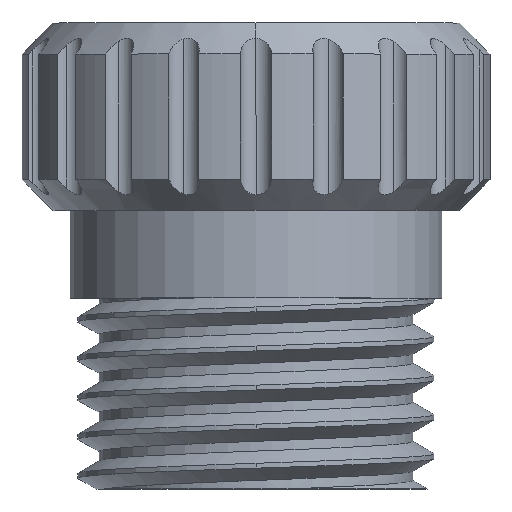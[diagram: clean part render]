
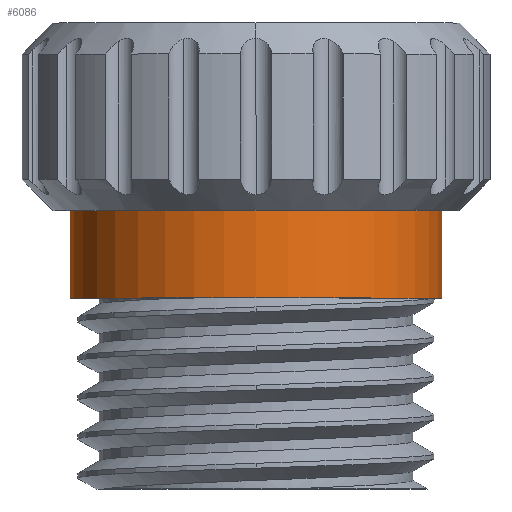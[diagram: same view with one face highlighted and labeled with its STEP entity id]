
A CAD part, top view. The second image highlights one B-rep face of the part: STEP entity #6086.
In plain terms, the highlighted cylindrical face has radius 7.556 mm (diameter 15.113 mm), a partial arc.
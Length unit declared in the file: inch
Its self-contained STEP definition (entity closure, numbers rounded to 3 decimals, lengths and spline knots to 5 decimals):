
#25 = DIRECTION ( 'NONE',  ( 0., -1., 0. ) ) ;
#44 = EDGE_CURVE ( 'NONE', #6907, #3247, #344, .T. ) ;
#344 = CIRCLE ( 'NONE', #1321, 0.2975 ) ;
#438 = CARTESIAN_POINT ( 'NONE',  ( 0., 0.305, -0.09256 ) ) ;
#463 = CARTESIAN_POINT ( 'NONE',  ( 0.16126, 0.305, -0.34256 ) ) ;
#691 = VECTOR ( 'NONE', #1452, 39.37008 ) ;
#1013 = ORIENTED_EDGE ( 'NONE', *, *, #2857, .T. ) ;
#1178 = DIRECTION ( 'NONE',  ( 0., 0., 1. ) ) ;
#1321 = AXIS2_PLACEMENT_3D ( 'NONE', #5092, #25, #1178 ) ;
#1392 = CARTESIAN_POINT ( 'NONE',  ( -0.16126, 0.305, -0.34256 ) ) ;
#1452 = DIRECTION ( 'NONE',  ( 0., 1., 0. ) ) ;
#1654 = LINE ( 'NONE', #2568, #1913 ) ;
#1792 = ORIENTED_EDGE ( 'NONE', *, *, #6013, .F. ) ;
#1909 = CARTESIAN_POINT ( 'NONE',  ( 0.16126, 0.445, -0.34256 ) ) ;
#1913 = VECTOR ( 'NONE', #3777, 39.37008 ) ;
#2059 = VERTEX_POINT ( 'NONE', #463 ) ;
#2178 = DIRECTION ( 'NONE',  ( 0., 0., 1. ) ) ;
#2227 = DIRECTION ( 'NONE',  ( 0., 0., -1. ) ) ;
#2568 = CARTESIAN_POINT ( 'NONE',  ( 0.16126, 0.305, -0.34256 ) ) ;
#2731 = AXIS2_PLACEMENT_3D ( 'NONE', #438, #7501, #2178 ) ;
#2857 = EDGE_CURVE ( 'NONE', #2059, #6907, #1654, .T. ) ;
#2866 = DIRECTION ( 'NONE',  ( 0., 1., 0. ) ) ;
#2942 = VERTEX_POINT ( 'NONE', #1392 ) ;
#3247 = VERTEX_POINT ( 'NONE', #6176 ) ;
#3777 = DIRECTION ( 'NONE',  ( 0., 1., 0. ) ) ;
#3871 = CYLINDRICAL_SURFACE ( 'NONE', #5873, 0.2975 ) ;
#4021 = CARTESIAN_POINT ( 'NONE',  ( 0., 0.305, -0.09256 ) ) ;
#4072 = FACE_OUTER_BOUND ( 'NONE', #6146, .T. ) ;
#4829 = ORIENTED_EDGE ( 'NONE', *, *, #44, .T. ) ;
#5092 = CARTESIAN_POINT ( 'NONE',  ( 0., 0.445, -0.09256 ) ) ;
#5873 = AXIS2_PLACEMENT_3D ( 'NONE', #4021, #2866, #2227 ) ;
#6013 = EDGE_CURVE ( 'NONE', #2059, #2942, #7162, .T. ) ;
#6086 = ADVANCED_FACE ( 'NONE', ( #4072 ), #3871, .T. ) ;
#6146 = EDGE_LOOP ( 'NONE', ( #4829, #7141, #1792, #1013 ) ) ;
#6176 = CARTESIAN_POINT ( 'NONE',  ( -0.16126, 0.445, -0.34256 ) ) ;
#6222 = LINE ( 'NONE', #6633, #691 ) ;
#6633 = CARTESIAN_POINT ( 'NONE',  ( -0.16126, 0.305, -0.34256 ) ) ;
#6907 = VERTEX_POINT ( 'NONE', #1909 ) ;
#7141 = ORIENTED_EDGE ( 'NONE', *, *, #7195, .F. ) ;
#7162 = CIRCLE ( 'NONE', #2731, 0.2975 ) ;
#7195 = EDGE_CURVE ( 'NONE', #2942, #3247, #6222, .T. ) ;
#7501 = DIRECTION ( 'NONE',  ( 0., -1., 0. ) ) ;
